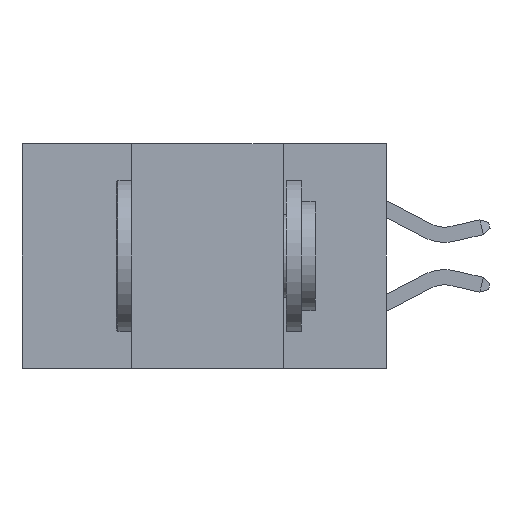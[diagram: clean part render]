
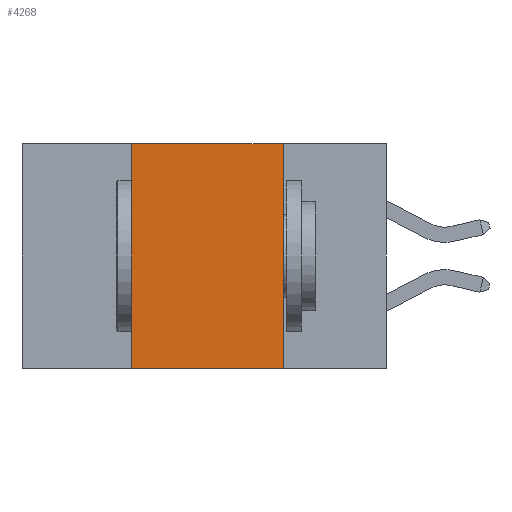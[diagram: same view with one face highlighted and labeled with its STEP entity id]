
A CAD part, left-side view. The second image highlights one B-rep face of the part: STEP entity #4268.
In plain terms, the highlighted planar face has unit normal (-1, 0, 0).
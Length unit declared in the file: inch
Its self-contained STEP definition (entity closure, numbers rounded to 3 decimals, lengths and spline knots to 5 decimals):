
#76 = LINE ( 'NONE', #10489, #3335 ) ;
#359 = CARTESIAN_POINT ( 'NONE',  ( 0., 0.6, 0. ) ) ;
#967 = VERTEX_POINT ( 'NONE', #6652 ) ;
#994 = AXIS2_PLACEMENT_3D ( 'NONE', #10935, #5884, #10991 ) ;
#1935 = EDGE_CURVE ( 'NONE', #3965, #6945, #8810, .T. ) ;
#2371 = ORIENTED_EDGE ( 'NONE', *, *, #1935, .F. ) ;
#2692 = DIRECTION ( 'NONE',  ( 0., 0., 1. ) ) ;
#2993 = DIRECTION ( 'NONE',  ( 0., -1., 0. ) ) ;
#3335 = VECTOR ( 'NONE', #4439, 39.37008 ) ;
#3358 = LINE ( 'NONE', #10184, #5104 ) ;
#3515 = EDGE_CURVE ( 'NONE', #967, #6789, #76, .T. ) ;
#3965 = VERTEX_POINT ( 'NONE', #7051 ) ;
#4268 = ADVANCED_FACE ( 'NONE', ( #9903 ), #7441, .F. ) ;
#4361 = EDGE_CURVE ( 'NONE', #967, #3965, #3358, .T. ) ;
#4439 = DIRECTION ( 'NONE',  ( 0., -1., 0. ) ) ;
#5104 = VECTOR ( 'NONE', #2692, 39.37008 ) ;
#5493 = CARTESIAN_POINT ( 'NONE',  ( 0., 0.17, -0.37 ) ) ;
#5498 = EDGE_CURVE ( 'NONE', #6945, #6789, #10596, .T. ) ;
#5834 = ORIENTED_EDGE ( 'NONE', *, *, #3515, .T. ) ;
#5884 = DIRECTION ( 'NONE',  ( 1., 0., 0. ) ) ;
#6277 = VECTOR ( 'NONE', #2993, 39.37008 ) ;
#6282 = CARTESIAN_POINT ( 'NONE',  ( 0., 0.17, 0. ) ) ;
#6652 = CARTESIAN_POINT ( 'NONE',  ( 0., 0.42, -0.37 ) ) ;
#6789 = VERTEX_POINT ( 'NONE', #9450 ) ;
#6945 = VERTEX_POINT ( 'NONE', #6282 ) ;
#7051 = CARTESIAN_POINT ( 'NONE',  ( 0., 0.42, 0. ) ) ;
#7167 = VECTOR ( 'NONE', #10879, 39.37008 ) ;
#7412 = ORIENTED_EDGE ( 'NONE', *, *, #4361, .F. ) ;
#7441 = PLANE ( 'NONE',  #994 ) ;
#8810 = LINE ( 'NONE', #359, #6277 ) ;
#8879 = ORIENTED_EDGE ( 'NONE', *, *, #5498, .F. ) ;
#9450 = CARTESIAN_POINT ( 'NONE',  ( 0., 0.17, -0.37 ) ) ;
#9903 = FACE_OUTER_BOUND ( 'NONE', #10161, .T. ) ;
#10161 = EDGE_LOOP ( 'NONE', ( #8879, #2371, #7412, #5834 ) ) ;
#10184 = CARTESIAN_POINT ( 'NONE',  ( 0., 0.42, -0.37 ) ) ;
#10489 = CARTESIAN_POINT ( 'NONE',  ( 0., 0.6, -0.37 ) ) ;
#10596 = LINE ( 'NONE', #5493, #7167 ) ;
#10879 = DIRECTION ( 'NONE',  ( 0., 0., -1. ) ) ;
#10935 = CARTESIAN_POINT ( 'NONE',  ( 0., 0.6, 0. ) ) ;
#10991 = DIRECTION ( 'NONE',  ( 0., 0., -1. ) ) ;
